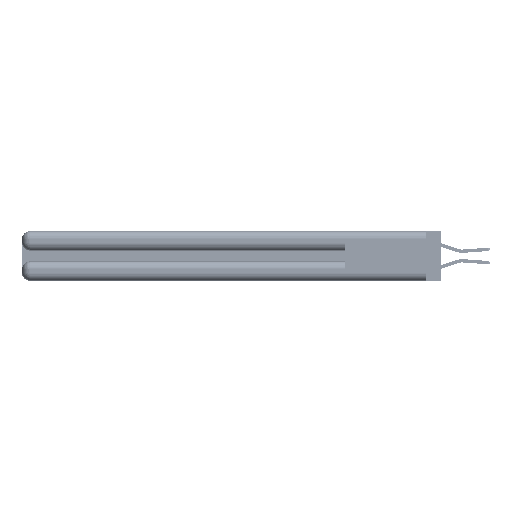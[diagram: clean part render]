
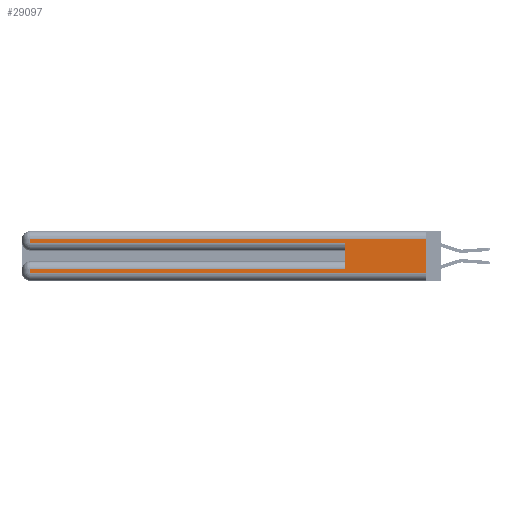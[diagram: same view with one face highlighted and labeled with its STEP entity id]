
A CAD part, left-side view. The second image highlights one B-rep face of the part: STEP entity #29097.
In plain terms, the highlighted planar face has unit normal (-1, 0, 0).
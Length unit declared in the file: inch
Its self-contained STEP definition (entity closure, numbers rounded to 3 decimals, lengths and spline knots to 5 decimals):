
#1978 = LINE ( 'NONE', #6137, #30231 ) ;
#3212 = CARTESIAN_POINT ( 'NONE',  ( 0., 0., 0.06 ) ) ;
#3246 = LINE ( 'NONE', #43486, #15713 ) ;
#3905 = VERTEX_POINT ( 'NONE', #8782 ) ;
#5802 = VERTEX_POINT ( 'NONE', #30219 ) ;
#5844 = DIRECTION ( 'NONE',  ( 0., 0., -1. ) ) ;
#6137 = CARTESIAN_POINT ( 'NONE',  ( 0., 2.94, 0.37 ) ) ;
#6608 = VECTOR ( 'NONE', #11188, 39.37008 ) ;
#7302 = VERTEX_POINT ( 'NONE', #15004 ) ;
#8250 = VERTEX_POINT ( 'NONE', #23339 ) ;
#8782 = CARTESIAN_POINT ( 'NONE',  ( 0., 2.94, 0.06 ) ) ;
#9011 = DIRECTION ( 'NONE',  ( 0., 0., -1. ) ) ;
#11188 = DIRECTION ( 'NONE',  ( 0., 1., 0. ) ) ;
#11251 = VECTOR ( 'NONE', #42348, 39.37008 ) ;
#12887 = EDGE_CURVE ( 'NONE', #48812, #7302, #17275, .T. ) ;
#13855 = DIRECTION ( 'NONE',  ( 0., 0., -1. ) ) ;
#14574 = EDGE_CURVE ( 'NONE', #3905, #22890, #34641, .T. ) ;
#15004 = CARTESIAN_POINT ( 'NONE',  ( 0., 2.94, 0.31 ) ) ;
#15713 = VECTOR ( 'NONE', #51767, 39.37008 ) ;
#15761 = DIRECTION ( 'NONE',  ( 0., 0., -1. ) ) ;
#17193 = EDGE_CURVE ( 'NONE', #29943, #5802, #21876, .T. ) ;
#17275 = LINE ( 'NONE', #23764, #6608 ) ;
#17356 = LINE ( 'NONE', #37661, #48127 ) ;
#19945 = DIRECTION ( 'NONE',  ( 0., -1., 0. ) ) ;
#20332 = EDGE_CURVE ( 'NONE', #5802, #3905, #22011, .T. ) ;
#21876 = LINE ( 'NONE', #47066, #11251 ) ;
#22011 = LINE ( 'NONE', #43849, #35250 ) ;
#22073 = CARTESIAN_POINT ( 'NONE',  ( 0., 0., 0.31 ) ) ;
#22890 = VERTEX_POINT ( 'NONE', #3212 ) ;
#23339 = CARTESIAN_POINT ( 'NONE',  ( 0., 0.6, 0.285 ) ) ;
#23764 = CARTESIAN_POINT ( 'NONE',  ( 0., 0., 0.31 ) ) ;
#24936 = DIRECTION ( 'NONE',  ( 1., 0., 0. ) ) ;
#26059 = EDGE_LOOP ( 'NONE', ( #26346, #37489, #35320, #42489, #26531, #48892, #33901, #36370 ) ) ;
#26346 = ORIENTED_EDGE ( 'NONE', *, *, #41312, .F. ) ;
#26531 = ORIENTED_EDGE ( 'NONE', *, *, #38101, .F. ) ;
#29097 = ADVANCED_FACE ( 'NONE', ( #46800 ), #40935, .F. ) ;
#29480 = EDGE_CURVE ( 'NONE', #33640, #8250, #30376, .T. ) ;
#29943 = VERTEX_POINT ( 'NONE', #37885 ) ;
#30219 = CARTESIAN_POINT ( 'NONE',  ( 0., 2.94, 0.085 ) ) ;
#30231 = VECTOR ( 'NONE', #13855, 39.37008 ) ;
#30239 = CARTESIAN_POINT ( 'NONE',  ( 0., 2.94, 0.285 ) ) ;
#30376 = LINE ( 'NONE', #35627, #31638 ) ;
#30731 = DIRECTION ( 'NONE',  ( 0., -1., 0. ) ) ;
#31638 = VECTOR ( 'NONE', #19945, 39.37008 ) ;
#33640 = VERTEX_POINT ( 'NONE', #30239 ) ;
#33901 = ORIENTED_EDGE ( 'NONE', *, *, #20332, .T. ) ;
#34641 = LINE ( 'NONE', #50584, #45348 ) ;
#35250 = VECTOR ( 'NONE', #15761, 39.37008 ) ;
#35320 = ORIENTED_EDGE ( 'NONE', *, *, #48785, .T. ) ;
#35627 = CARTESIAN_POINT ( 'NONE',  ( 0., 0., 0.285 ) ) ;
#36370 = ORIENTED_EDGE ( 'NONE', *, *, #14574, .T. ) ;
#37489 = ORIENTED_EDGE ( 'NONE', *, *, #12887, .T. ) ;
#37661 = CARTESIAN_POINT ( 'NONE',  ( 0., 0., 0.37 ) ) ;
#37885 = CARTESIAN_POINT ( 'NONE',  ( 0., 0.6, 0.085 ) ) ;
#38101 = EDGE_CURVE ( 'NONE', #29943, #8250, #3246, .T. ) ;
#40935 = PLANE ( 'NONE',  #50430 ) ;
#41312 = EDGE_CURVE ( 'NONE', #48812, #22890, #17356, .T. ) ;
#42348 = DIRECTION ( 'NONE',  ( 0., 1., 0. ) ) ;
#42489 = ORIENTED_EDGE ( 'NONE', *, *, #29480, .T. ) ;
#43486 = CARTESIAN_POINT ( 'NONE',  ( 0., 0.6, 0.145 ) ) ;
#43849 = CARTESIAN_POINT ( 'NONE',  ( 0., 2.94, 0.37 ) ) ;
#45348 = VECTOR ( 'NONE', #30731, 39.37008 ) ;
#46800 = FACE_OUTER_BOUND ( 'NONE', #26059, .T. ) ;
#47066 = CARTESIAN_POINT ( 'NONE',  ( 0., 0., 0.085 ) ) ;
#48127 = VECTOR ( 'NONE', #5844, 39.37008 ) ;
#48785 = EDGE_CURVE ( 'NONE', #7302, #33640, #1978, .T. ) ;
#48812 = VERTEX_POINT ( 'NONE', #22073 ) ;
#48892 = ORIENTED_EDGE ( 'NONE', *, *, #17193, .T. ) ;
#48984 = CARTESIAN_POINT ( 'NONE',  ( 0., 0., 0.37 ) ) ;
#50430 = AXIS2_PLACEMENT_3D ( 'NONE', #48984, #24936, #9011 ) ;
#50584 = CARTESIAN_POINT ( 'NONE',  ( 0., 0., 0.06 ) ) ;
#51767 = DIRECTION ( 'NONE',  ( 0., 0., 1. ) ) ;
